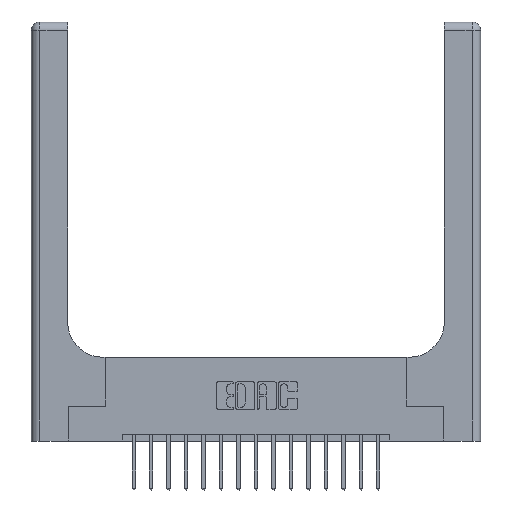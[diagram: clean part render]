
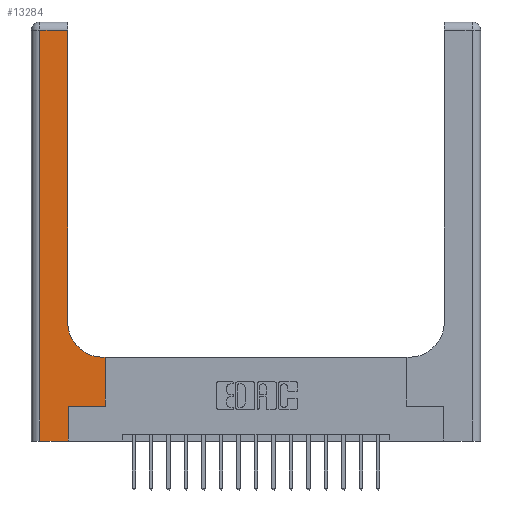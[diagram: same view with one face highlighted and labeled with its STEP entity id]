
A CAD part, top view. The second image highlights one B-rep face of the part: STEP entity #13284.
In plain terms, the highlighted planar face has unit normal (0, 0, 1).
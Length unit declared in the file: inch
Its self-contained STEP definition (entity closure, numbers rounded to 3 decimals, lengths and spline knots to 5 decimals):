
#112 = DIRECTION ( 'NONE',  ( 0., -1., 0. ) ) ;
#135 = VERTEX_POINT ( 'NONE', #18526 ) ;
#394 = VERTEX_POINT ( 'NONE', #6954 ) ;
#599 = DIRECTION ( 'NONE',  ( -1., 0., 0. ) ) ;
#664 = AXIS2_PLACEMENT_3D ( 'NONE', #13997, #1125, #13940 ) ;
#746 = VERTEX_POINT ( 'NONE', #2202 ) ;
#768 = VECTOR ( 'NONE', #17180, 39.37008 ) ;
#788 = EDGE_CURVE ( 'NONE', #8897, #2695, #5057, .T. ) ;
#1034 = VECTOR ( 'NONE', #12632, 39.37008 ) ;
#1125 = DIRECTION ( 'NONE',  ( 0., 0., -1. ) ) ;
#1452 = VERTEX_POINT ( 'NONE', #2022 ) ;
#1845 = LINE ( 'NONE', #15121, #11966 ) ;
#2022 = CARTESIAN_POINT ( 'NONE',  ( 0.26, 0.85, 0.37 ) ) ;
#2095 = DIRECTION ( 'NONE',  ( 1., 0., 0. ) ) ;
#2141 = EDGE_CURVE ( 'NONE', #746, #9367, #13070, .T. ) ;
#2202 = CARTESIAN_POINT ( 'NONE',  ( 0.265, 0., 0.37 ) ) ;
#2695 = VERTEX_POINT ( 'NONE', #4765 ) ;
#2934 = DIRECTION ( 'NONE',  ( 1., 0., 0. ) ) ;
#2995 = DIRECTION ( 'NONE',  ( 1., 0., 0. ) ) ;
#3062 = DIRECTION ( 'NONE',  ( 0., 0., -1. ) ) ;
#3328 = ORIENTED_EDGE ( 'NONE', *, *, #16985, .T. ) ;
#3591 = DIRECTION ( 'NONE',  ( 0., 1., 0. ) ) ;
#3602 = ORIENTED_EDGE ( 'NONE', *, *, #11428, .T. ) ;
#4087 = CARTESIAN_POINT ( 'NONE',  ( 0.26, 3., 0.37 ) ) ;
#4217 = ORIENTED_EDGE ( 'NONE', *, *, #788, .T. ) ;
#4272 = CARTESIAN_POINT ( 'NONE',  ( 0.26, 2.94, 0.37 ) ) ;
#4765 = CARTESIAN_POINT ( 'NONE',  ( 0.06, 2.94, 0.37 ) ) ;
#4797 = ORIENTED_EDGE ( 'NONE', *, *, #17132, .T. ) ;
#5057 = LINE ( 'NONE', #15047, #15171 ) ;
#5275 = LINE ( 'NONE', #9906, #768 ) ;
#5928 = LINE ( 'NONE', #10742, #7280 ) ;
#6145 = EDGE_CURVE ( 'NONE', #394, #135, #5275, .T. ) ;
#6272 = FACE_OUTER_BOUND ( 'NONE', #13176, .T. ) ;
#6954 = CARTESIAN_POINT ( 'NONE',  ( 0.528, 0.25, 0.37 ) ) ;
#6955 = AXIS2_PLACEMENT_3D ( 'NONE', #8852, #3062, #2995 ) ;
#7053 = EDGE_CURVE ( 'NONE', #135, #18255, #1845, .T. ) ;
#7280 = VECTOR ( 'NONE', #2095, 39.37008 ) ;
#7446 = VECTOR ( 'NONE', #3591, 39.37008 ) ;
#7516 = EDGE_CURVE ( 'NONE', #9367, #394, #5928, .T. ) ;
#7561 = CIRCLE ( 'NONE', #6955, 0.25 ) ;
#8262 = ORIENTED_EDGE ( 'NONE', *, *, #14750, .T. ) ;
#8592 = CARTESIAN_POINT ( 'NONE',  ( 0.06, 0., 0.37 ) ) ;
#8761 = ORIENTED_EDGE ( 'NONE', *, *, #7516, .T. ) ;
#8852 = CARTESIAN_POINT ( 'NONE',  ( 0.51, 0.85, 0.37 ) ) ;
#8897 = VERTEX_POINT ( 'NONE', #4272 ) ;
#9122 = LINE ( 'NONE', #4087, #1034 ) ;
#9238 = VECTOR ( 'NONE', #2934, 39.37008 ) ;
#9367 = VERTEX_POINT ( 'NONE', #11418 ) ;
#9519 = DIRECTION ( 'NONE',  ( -1., 0., 0. ) ) ;
#9906 = CARTESIAN_POINT ( 'NONE',  ( 0.528, 0.25, 0.37 ) ) ;
#10742 = CARTESIAN_POINT ( 'NONE',  ( 0.265, 0.25, 0.37 ) ) ;
#11411 = CARTESIAN_POINT ( 'NONE',  ( 0.51, 0.6, 0.37 ) ) ;
#11418 = CARTESIAN_POINT ( 'NONE',  ( 0.265, 0.25, 0.37 ) ) ;
#11428 = EDGE_CURVE ( 'NONE', #18163, #746, #13734, .T. ) ;
#11804 = LINE ( 'NONE', #17357, #13819 ) ;
#11966 = VECTOR ( 'NONE', #9519, 39.37008 ) ;
#12632 = DIRECTION ( 'NONE',  ( 0., 1., 0. ) ) ;
#13070 = LINE ( 'NONE', #17924, #7446 ) ;
#13176 = EDGE_LOOP ( 'NONE', ( #3328, #4217, #4797, #3602, #15709, #8761, #17049, #15119, #8262 ) ) ;
#13284 = ADVANCED_FACE ( 'NONE', ( #6272 ), #18416, .F. ) ;
#13734 = LINE ( 'NONE', #14195, #9238 ) ;
#13819 = VECTOR ( 'NONE', #112, 39.37008 ) ;
#13940 = DIRECTION ( 'NONE',  ( -1., 0., 0. ) ) ;
#13997 = CARTESIAN_POINT ( 'NONE',  ( 0., 3., 0.37 ) ) ;
#14195 = CARTESIAN_POINT ( 'NONE',  ( 0., 0., 0.37 ) ) ;
#14750 = EDGE_CURVE ( 'NONE', #18255, #1452, #7561, .T. ) ;
#15047 = CARTESIAN_POINT ( 'NONE',  ( 0., 2.94, 0.37 ) ) ;
#15119 = ORIENTED_EDGE ( 'NONE', *, *, #7053, .T. ) ;
#15121 = CARTESIAN_POINT ( 'NONE',  ( 0.26, 0.6, 0.37 ) ) ;
#15171 = VECTOR ( 'NONE', #599, 39.37008 ) ;
#15709 = ORIENTED_EDGE ( 'NONE', *, *, #2141, .T. ) ;
#16985 = EDGE_CURVE ( 'NONE', #1452, #8897, #9122, .T. ) ;
#17049 = ORIENTED_EDGE ( 'NONE', *, *, #6145, .T. ) ;
#17132 = EDGE_CURVE ( 'NONE', #2695, #18163, #11804, .T. ) ;
#17180 = DIRECTION ( 'NONE',  ( 0., 1., 0. ) ) ;
#17357 = CARTESIAN_POINT ( 'NONE',  ( 0.06, 3., 0.37 ) ) ;
#17924 = CARTESIAN_POINT ( 'NONE',  ( 0.265, 0., 0.37 ) ) ;
#18163 = VERTEX_POINT ( 'NONE', #8592 ) ;
#18255 = VERTEX_POINT ( 'NONE', #11411 ) ;
#18416 = PLANE ( 'NONE',  #664 ) ;
#18526 = CARTESIAN_POINT ( 'NONE',  ( 0.528, 0.6, 0.37 ) ) ;
